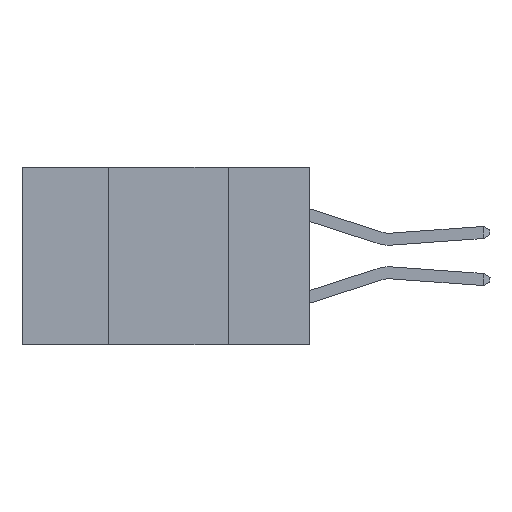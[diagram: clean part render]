
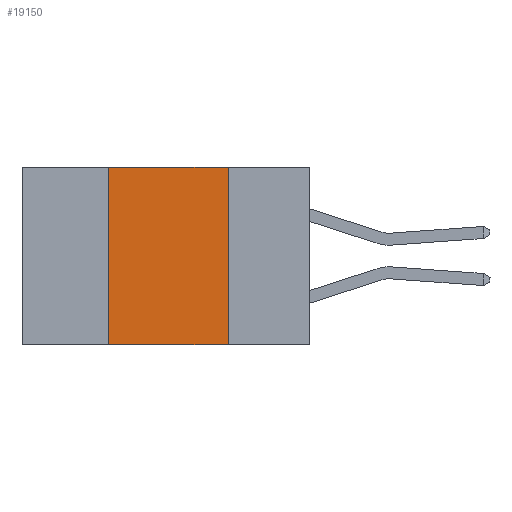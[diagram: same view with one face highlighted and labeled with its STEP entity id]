
A CAD part, left-side view. The second image highlights one B-rep face of the part: STEP entity #19150.
In plain terms, the highlighted planar face has unit normal (-1, 0, 0).
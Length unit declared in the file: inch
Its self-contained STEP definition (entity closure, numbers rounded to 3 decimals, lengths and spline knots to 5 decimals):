
#527 = ORIENTED_EDGE ( 'NONE', *, *, #17910, .F. ) ;
#1465 = VERTEX_POINT ( 'NONE', #19954 ) ;
#3394 = AXIS2_PLACEMENT_3D ( 'NONE', #19296, #8975, #21013 ) ;
#3550 = LINE ( 'NONE', #9096, #19203 ) ;
#3894 = ORIENTED_EDGE ( 'NONE', *, *, #19865, .T. ) ;
#4958 = CARTESIAN_POINT ( 'NONE',  ( 0., 0.42, -0.37 ) ) ;
#5494 = PLANE ( 'NONE',  #3394 ) ;
#5804 = VECTOR ( 'NONE', #12956, 39.37008 ) ;
#7120 = VERTEX_POINT ( 'NONE', #4958 ) ;
#8150 = ORIENTED_EDGE ( 'NONE', *, *, #17906, .F. ) ;
#8975 = DIRECTION ( 'NONE',  ( 1., 0., 0. ) ) ;
#9096 = CARTESIAN_POINT ( 'NONE',  ( 0., 0.6, -0.37 ) ) ;
#9119 = ORIENTED_EDGE ( 'NONE', *, *, #18743, .F. ) ;
#9415 = CARTESIAN_POINT ( 'NONE',  ( 0., 0.17, -0.37 ) ) ;
#10850 = DIRECTION ( 'NONE',  ( 0., -1., 0. ) ) ;
#10886 = VERTEX_POINT ( 'NONE', #9415 ) ;
#11078 = EDGE_LOOP ( 'NONE', ( #527, #9119, #8150, #3894 ) ) ;
#12896 = CARTESIAN_POINT ( 'NONE',  ( 0., 0.42, 0. ) ) ;
#12956 = DIRECTION ( 'NONE',  ( 0., 0., -1. ) ) ;
#13400 = LINE ( 'NONE', #12896, #15017 ) ;
#14162 = LINE ( 'NONE', #20054, #21407 ) ;
#14188 = VERTEX_POINT ( 'NONE', #20711 ) ;
#14478 = LINE ( 'NONE', #19931, #5804 ) ;
#15017 = VECTOR ( 'NONE', #21448, 39.37008 ) ;
#17636 = FACE_OUTER_BOUND ( 'NONE', #11078, .T. ) ;
#17906 = EDGE_CURVE ( 'NONE', #7120, #14188, #13400, .T. ) ;
#17910 = EDGE_CURVE ( 'NONE', #1465, #10886, #14478, .T. ) ;
#18743 = EDGE_CURVE ( 'NONE', #14188, #1465, #14162, .T. ) ;
#19150 = ADVANCED_FACE ( 'NONE', ( #17636 ), #5494, .F. ) ;
#19203 = VECTOR ( 'NONE', #10850, 39.37008 ) ;
#19296 = CARTESIAN_POINT ( 'NONE',  ( 0., 0.6, 0. ) ) ;
#19865 = EDGE_CURVE ( 'NONE', #7120, #10886, #3550, .T. ) ;
#19931 = CARTESIAN_POINT ( 'NONE',  ( 0., 0.17, 0. ) ) ;
#19954 = CARTESIAN_POINT ( 'NONE',  ( 0., 0.17, 0. ) ) ;
#20054 = CARTESIAN_POINT ( 'NONE',  ( 0., 0.6, 0. ) ) ;
#20711 = CARTESIAN_POINT ( 'NONE',  ( 0., 0.42, 0. ) ) ;
#21013 = DIRECTION ( 'NONE',  ( 0., 0., -1. ) ) ;
#21407 = VECTOR ( 'NONE', #21961, 39.37008 ) ;
#21448 = DIRECTION ( 'NONE',  ( 0., 0., 1. ) ) ;
#21961 = DIRECTION ( 'NONE',  ( 0., -1., 0. ) ) ;
